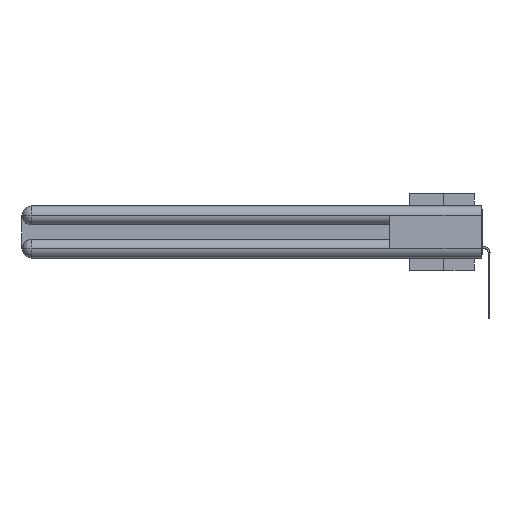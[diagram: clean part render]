
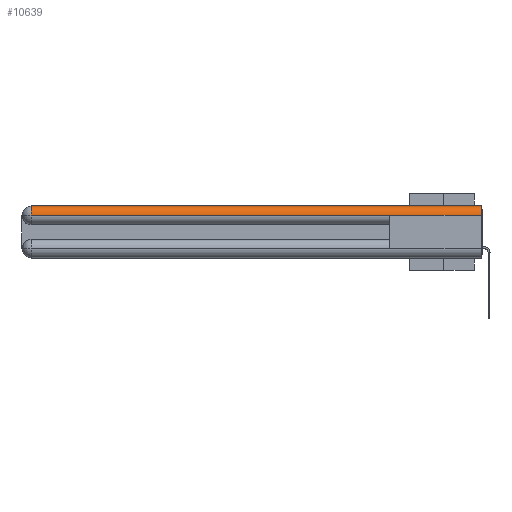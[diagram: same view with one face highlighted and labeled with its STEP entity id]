
A CAD part, left-side view. The second image highlights one B-rep face of the part: STEP entity #10639.
In plain terms, the highlighted cylindrical face has radius 1.562 mm (diameter 3.124 mm), a partial arc.
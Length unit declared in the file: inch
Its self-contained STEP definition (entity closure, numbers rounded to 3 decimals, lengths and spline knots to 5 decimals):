
#266 = EDGE_CURVE ( 'NONE', #15106, #14293, #11613, .T. ) ;
#1338 = AXIS2_PLACEMENT_3D ( 'NONE', #9662, #20039, #17485 ) ;
#2039 = EDGE_CURVE ( 'NONE', #9599, #10856, #16991, .T. ) ;
#2484 = ORIENTED_EDGE ( 'NONE', *, *, #8316, .T. ) ;
#2495 = VECTOR ( 'NONE', #29990, 39.37008 ) ;
#2584 = AXIS2_PLACEMENT_3D ( 'NONE', #8333, #18539, #18021 ) ;
#2742 = CYLINDRICAL_SURFACE ( 'NONE', #2584, 0.0615 ) ;
#3229 = DIRECTION ( 'NONE',  ( 0., -1., 0. ) ) ;
#3291 = EDGE_CURVE ( 'NONE', #14293, #20978, #32752, .T. ) ;
#4162 = CARTESIAN_POINT ( 'NONE',  ( 0., 3., -0.0615 ) ) ;
#4395 = CARTESIAN_POINT ( 'NONE',  ( 0., 2.94, -0.0615 ) ) ;
#6537 = DIRECTION ( 'NONE',  ( 0., -1., 0. ) ) ;
#6833 = CARTESIAN_POINT ( 'NONE',  ( 0.0615, 0., 0. ) ) ;
#7613 = EDGE_CURVE ( 'NONE', #9599, #15106, #17533, .T. ) ;
#8316 = EDGE_CURVE ( 'NONE', #10856, #20978, #11526, .T. ) ;
#8333 = CARTESIAN_POINT ( 'NONE',  ( 0.0615, 0., -0.0615 ) ) ;
#9599 = VERTEX_POINT ( 'NONE', #13901 ) ;
#9662 = CARTESIAN_POINT ( 'NONE',  ( 0.0615, 0., -0.0615 ) ) ;
#10639 = ADVANCED_FACE ( 'NONE', ( #26203 ), #2742, .T. ) ;
#10856 = VERTEX_POINT ( 'NONE', #4395 ) ;
#11219 = VECTOR ( 'NONE', #3229, 39.37008 ) ;
#11526 = LINE ( 'NONE', #16605, #11219 ) ;
#11613 = CIRCLE ( 'NONE', #1338, 0.0615 ) ;
#13353 = ORIENTED_EDGE ( 'NONE', *, *, #7613, .F. ) ;
#13744 = AXIS2_PLACEMENT_3D ( 'NONE', #30169, #6537, #22189 ) ;
#13901 = CARTESIAN_POINT ( 'NONE',  ( 0.0615, 2.94, 0. ) ) ;
#14293 = VERTEX_POINT ( 'NONE', #27321 ) ;
#15106 = VERTEX_POINT ( 'NONE', #19687 ) ;
#15888 = ORIENTED_EDGE ( 'NONE', *, *, #2039, .T. ) ;
#16605 = CARTESIAN_POINT ( 'NONE',  ( 0., 3., -0.0615 ) ) ;
#16991 = CIRCLE ( 'NONE', #13744, 0.0615 ) ;
#17485 = DIRECTION ( 'NONE',  ( 1., 0., 0. ) ) ;
#17533 = LINE ( 'NONE', #6833, #2495 ) ;
#18021 = DIRECTION ( 'NONE',  ( 0., 0., 1. ) ) ;
#18539 = DIRECTION ( 'NONE',  ( 0., 1., 0. ) ) ;
#19469 = DIRECTION ( 'NONE',  ( 0., 1., 0. ) ) ;
#19687 = CARTESIAN_POINT ( 'NONE',  ( 0.0615, 0., 0. ) ) ;
#20039 = DIRECTION ( 'NONE',  ( 0., -1., 0. ) ) ;
#20978 = VERTEX_POINT ( 'NONE', #22967 ) ;
#22189 = DIRECTION ( 'NONE',  ( 0., 0., 1. ) ) ;
#22852 = EDGE_LOOP ( 'NONE', ( #13353, #15888, #2484, #30670, #25472 ) ) ;
#22967 = CARTESIAN_POINT ( 'NONE',  ( 0., 0.6, -0.0615 ) ) ;
#25472 = ORIENTED_EDGE ( 'NONE', *, *, #266, .F. ) ;
#26203 = FACE_OUTER_BOUND ( 'NONE', #22852, .T. ) ;
#27321 = CARTESIAN_POINT ( 'NONE',  ( 0., 0., -0.0615 ) ) ;
#27878 = VECTOR ( 'NONE', #19469, 39.37008 ) ;
#29990 = DIRECTION ( 'NONE',  ( 0., -1., 0. ) ) ;
#30169 = CARTESIAN_POINT ( 'NONE',  ( 0.0615, 2.94, -0.0615 ) ) ;
#30670 = ORIENTED_EDGE ( 'NONE', *, *, #3291, .F. ) ;
#32752 = LINE ( 'NONE', #4162, #27878 ) ;
